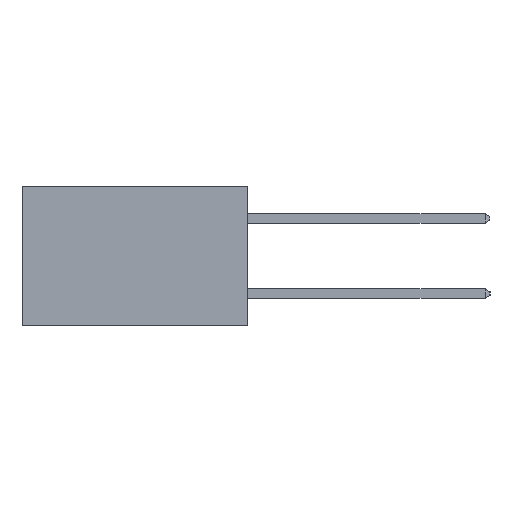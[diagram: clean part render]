
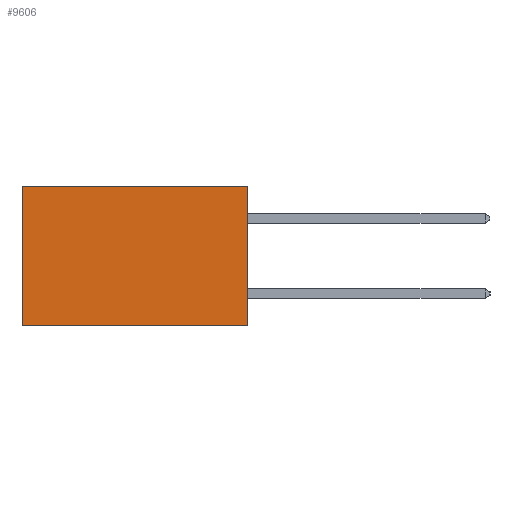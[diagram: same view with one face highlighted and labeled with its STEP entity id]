
A CAD part, left-side view. The second image highlights one B-rep face of the part: STEP entity #9606.
In plain terms, the highlighted planar face has unit normal (-1, 0, 0).
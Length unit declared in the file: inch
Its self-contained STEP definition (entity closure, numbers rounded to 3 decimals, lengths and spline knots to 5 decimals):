
#1018 = CARTESIAN_POINT ( 'NONE',  ( 0.2615, 0., -0.37 ) ) ;
#1256 = CARTESIAN_POINT ( 'NONE',  ( 0.2615, 0., -0.37 ) ) ;
#1432 = DIRECTION ( 'NONE',  ( 0., 1., 0. ) ) ;
#1667 = EDGE_CURVE ( 'NONE', #6939, #16476, #5666, .T. ) ;
#1770 = CARTESIAN_POINT ( 'NONE',  ( 0.2615, 0., 0. ) ) ;
#1780 = ORIENTED_EDGE ( 'NONE', *, *, #6992, .F. ) ;
#1888 = VECTOR ( 'NONE', #14316, 39.37008 ) ;
#2237 = EDGE_CURVE ( 'NONE', #6939, #5255, #17194, .T. ) ;
#2598 = FACE_OUTER_BOUND ( 'NONE', #7986, .T. ) ;
#2674 = EDGE_CURVE ( 'NONE', #16476, #5440, #11763, .T. ) ;
#2766 = DIRECTION ( 'NONE',  ( 1., 0., 0. ) ) ;
#2980 = LINE ( 'NONE', #1018, #10018 ) ;
#5144 = ORIENTED_EDGE ( 'NONE', *, *, #2674, .T. ) ;
#5255 = VERTEX_POINT ( 'NONE', #14070 ) ;
#5440 = VERTEX_POINT ( 'NONE', #5965 ) ;
#5666 = LINE ( 'NONE', #14471, #1888 ) ;
#5965 = CARTESIAN_POINT ( 'NONE',  ( 0.2615, 0.6, -0.37 ) ) ;
#6739 = VECTOR ( 'NONE', #9247, 39.37008 ) ;
#6939 = VERTEX_POINT ( 'NONE', #1770 ) ;
#6992 = EDGE_CURVE ( 'NONE', #5255, #5440, #2980, .T. ) ;
#7795 = DIRECTION ( 'NONE',  ( 0., 0., -1. ) ) ;
#7986 = EDGE_LOOP ( 'NONE', ( #5144, #1780, #13437, #15968 ) ) ;
#8042 = VECTOR ( 'NONE', #7795, 39.37008 ) ;
#9247 = DIRECTION ( 'NONE',  ( 0., 0., -1. ) ) ;
#9558 = CARTESIAN_POINT ( 'NONE',  ( 0.2615, 0., -0.37 ) ) ;
#9606 = ADVANCED_FACE ( 'NONE', ( #2598 ), #17839, .F. ) ;
#9933 = CARTESIAN_POINT ( 'NONE',  ( 0.2615, 0.6, -0.37 ) ) ;
#10018 = VECTOR ( 'NONE', #1432, 39.37008 ) ;
#11763 = LINE ( 'NONE', #9933, #8042 ) ;
#12588 = DIRECTION ( 'NONE',  ( 0., 0., -1. ) ) ;
#13437 = ORIENTED_EDGE ( 'NONE', *, *, #2237, .F. ) ;
#14070 = CARTESIAN_POINT ( 'NONE',  ( 0.2615, 0., -0.37 ) ) ;
#14316 = DIRECTION ( 'NONE',  ( 0., 1., 0. ) ) ;
#14471 = CARTESIAN_POINT ( 'NONE',  ( 0.2615, 0., 0. ) ) ;
#15968 = ORIENTED_EDGE ( 'NONE', *, *, #1667, .T. ) ;
#16246 = AXIS2_PLACEMENT_3D ( 'NONE', #1256, #2766, #12588 ) ;
#16476 = VERTEX_POINT ( 'NONE', #17868 ) ;
#17194 = LINE ( 'NONE', #9558, #6739 ) ;
#17839 = PLANE ( 'NONE',  #16246 ) ;
#17868 = CARTESIAN_POINT ( 'NONE',  ( 0.2615, 0.6, 0. ) ) ;
